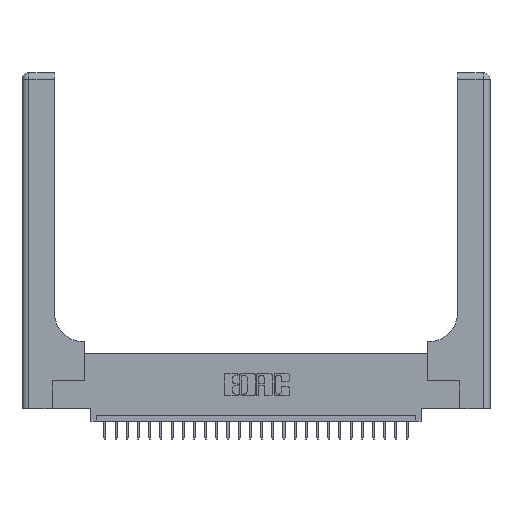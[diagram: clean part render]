
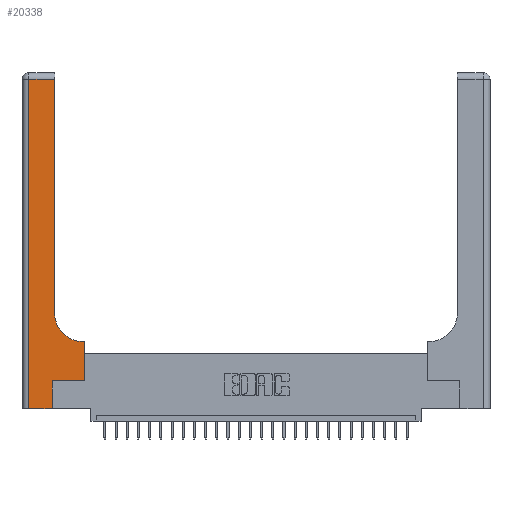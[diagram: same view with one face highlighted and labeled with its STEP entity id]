
A CAD part, top view. The second image highlights one B-rep face of the part: STEP entity #20338.
In plain terms, the highlighted planar face has unit normal (0, 0, 1).
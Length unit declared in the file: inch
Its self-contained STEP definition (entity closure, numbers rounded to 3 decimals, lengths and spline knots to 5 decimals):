
#258 = CARTESIAN_POINT ( 'NONE',  ( 0.5585, 0.25, 0.37 ) ) ;
#1045 = CARTESIAN_POINT ( 'NONE',  ( 0.5585, 0.6, 0.37 ) ) ;
#1261 = CARTESIAN_POINT ( 'NONE',  ( 0.269, 0.25, 0.37 ) ) ;
#1335 = VERTEX_POINT ( 'NONE', #24731 ) ;
#2119 = CARTESIAN_POINT ( 'NONE',  ( 0.2915, 0.85, 0.37 ) ) ;
#2294 = ORIENTED_EDGE ( 'NONE', *, *, #9215, .T. ) ;
#3008 = VECTOR ( 'NONE', #10347, 39.37008 ) ;
#3216 = EDGE_CURVE ( 'NONE', #3596, #8668, #10629, .T. ) ;
#3326 = LINE ( 'NONE', #22756, #3008 ) ;
#3596 = VERTEX_POINT ( 'NONE', #1261 ) ;
#3977 = LINE ( 'NONE', #7990, #26588 ) ;
#4414 = EDGE_CURVE ( 'NONE', #8713, #25557, #27683, .T. ) ;
#4685 = LINE ( 'NONE', #258, #14304 ) ;
#5074 = DIRECTION ( 'NONE',  ( -1., 0., 0. ) ) ;
#5309 = VERTEX_POINT ( 'NONE', #7307 ) ;
#5409 = DIRECTION ( 'NONE',  ( -1., 0., 0. ) ) ;
#5923 = VERTEX_POINT ( 'NONE', #1045 ) ;
#6741 = AXIS2_PLACEMENT_3D ( 'NONE', #27439, #24161, #5409 ) ;
#7307 = CARTESIAN_POINT ( 'NONE',  ( 0.06, 2.94, 0.37 ) ) ;
#7792 = DIRECTION ( 'NONE',  ( 0., 0., -1. ) ) ;
#7990 = CARTESIAN_POINT ( 'NONE',  ( 0.2915, 0.6, 0.37 ) ) ;
#8147 = EDGE_CURVE ( 'NONE', #5309, #8713, #3326, .T. ) ;
#8668 = VERTEX_POINT ( 'NONE', #18978 ) ;
#8713 = VERTEX_POINT ( 'NONE', #20992 ) ;
#8827 = VERTEX_POINT ( 'NONE', #2119 ) ;
#9215 = EDGE_CURVE ( 'NONE', #25557, #3596, #11187, .T. ) ;
#9804 = DIRECTION ( 'NONE',  ( -1., 0., 0. ) ) ;
#10347 = DIRECTION ( 'NONE',  ( 0., -1., 0. ) ) ;
#10629 = LINE ( 'NONE', #18517, #24650 ) ;
#10877 = CARTESIAN_POINT ( 'NONE',  ( 0.269, 0., 0.37 ) ) ;
#10990 = ORIENTED_EDGE ( 'NONE', *, *, #15712, .T. ) ;
#11187 = LINE ( 'NONE', #12382, #22143 ) ;
#12109 = CARTESIAN_POINT ( 'NONE',  ( 0.5415, 0.85, 0.37 ) ) ;
#12382 = CARTESIAN_POINT ( 'NONE',  ( 0.269, 0., 0.37 ) ) ;
#12773 = ORIENTED_EDGE ( 'NONE', *, *, #23995, .T. ) ;
#13417 = AXIS2_PLACEMENT_3D ( 'NONE', #12109, #7792, #18695 ) ;
#13629 = VECTOR ( 'NONE', #5074, 39.37008 ) ;
#13773 = DIRECTION ( 'NONE',  ( 0., 1., 0. ) ) ;
#14304 = VECTOR ( 'NONE', #15375, 39.37008 ) ;
#15375 = DIRECTION ( 'NONE',  ( 0., 1., 0. ) ) ;
#15384 = ORIENTED_EDGE ( 'NONE', *, *, #23703, .T. ) ;
#15620 = CARTESIAN_POINT ( 'NONE',  ( 0.5415, 0.6, 0.37 ) ) ;
#15712 = EDGE_CURVE ( 'NONE', #8827, #1335, #26741, .T. ) ;
#16199 = CARTESIAN_POINT ( 'NONE',  ( 0., 2.94, 0.37 ) ) ;
#16302 = PLANE ( 'NONE',  #6741 ) ;
#17892 = CARTESIAN_POINT ( 'NONE',  ( 0.2915, 3., 0.37 ) ) ;
#18517 = CARTESIAN_POINT ( 'NONE',  ( 0.269, 0.25, 0.37 ) ) ;
#18695 = DIRECTION ( 'NONE',  ( 1., 0., 0. ) ) ;
#18790 = DIRECTION ( 'NONE',  ( 1., 0., 0. ) ) ;
#18978 = CARTESIAN_POINT ( 'NONE',  ( 0.5585, 0.25, 0.37 ) ) ;
#20338 = ADVANCED_FACE ( 'NONE', ( #23751 ), #16302, .F. ) ;
#20479 = ORIENTED_EDGE ( 'NONE', *, *, #4414, .T. ) ;
#20744 = ORIENTED_EDGE ( 'NONE', *, *, #8147, .T. ) ;
#20992 = CARTESIAN_POINT ( 'NONE',  ( 0.06, 0., 0.37 ) ) ;
#21258 = DIRECTION ( 'NONE',  ( 0., 1., 0. ) ) ;
#21665 = ORIENTED_EDGE ( 'NONE', *, *, #23145, .T. ) ;
#21755 = DIRECTION ( 'NONE',  ( 1., 0., 0. ) ) ;
#22143 = VECTOR ( 'NONE', #21258, 39.37008 ) ;
#22756 = CARTESIAN_POINT ( 'NONE',  ( 0.06, 3., 0.37 ) ) ;
#23145 = EDGE_CURVE ( 'NONE', #1335, #5309, #23916, .T. ) ;
#23703 = EDGE_CURVE ( 'NONE', #8668, #5923, #4685, .T. ) ;
#23751 = FACE_OUTER_BOUND ( 'NONE', #25639, .T. ) ;
#23904 = EDGE_CURVE ( 'NONE', #24402, #8827, #25920, .T. ) ;
#23916 = LINE ( 'NONE', #16199, #13629 ) ;
#23926 = VECTOR ( 'NONE', #21755, 39.37008 ) ;
#23930 = ORIENTED_EDGE ( 'NONE', *, *, #23904, .T. ) ;
#23995 = EDGE_CURVE ( 'NONE', #5923, #24402, #3977, .T. ) ;
#24161 = DIRECTION ( 'NONE',  ( 0., 0., -1. ) ) ;
#24402 = VERTEX_POINT ( 'NONE', #15620 ) ;
#24650 = VECTOR ( 'NONE', #18790, 39.37008 ) ;
#24731 = CARTESIAN_POINT ( 'NONE',  ( 0.2915, 2.94, 0.37 ) ) ;
#25557 = VERTEX_POINT ( 'NONE', #10877 ) ;
#25639 = EDGE_LOOP ( 'NONE', ( #10990, #21665, #20744, #20479, #2294, #26960, #15384, #12773, #23930 ) ) ;
#25751 = VECTOR ( 'NONE', #13773, 39.37008 ) ;
#25805 = CARTESIAN_POINT ( 'NONE',  ( 0., 0., 0.37 ) ) ;
#25920 = CIRCLE ( 'NONE', #13417, 0.25 ) ;
#26588 = VECTOR ( 'NONE', #9804, 39.37008 ) ;
#26741 = LINE ( 'NONE', #17892, #25751 ) ;
#26960 = ORIENTED_EDGE ( 'NONE', *, *, #3216, .T. ) ;
#27439 = CARTESIAN_POINT ( 'NONE',  ( 0., 3., 0.37 ) ) ;
#27683 = LINE ( 'NONE', #25805, #23926 ) ;
